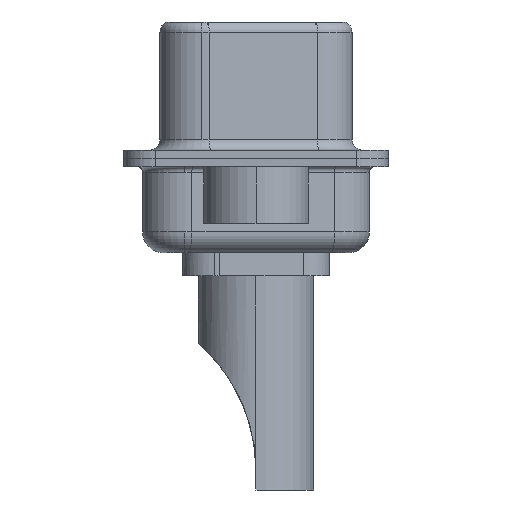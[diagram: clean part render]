
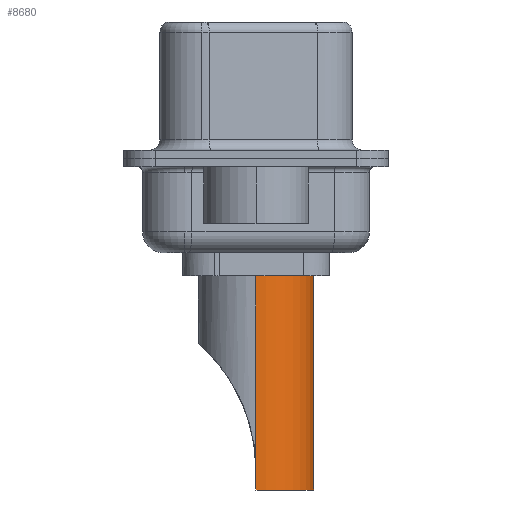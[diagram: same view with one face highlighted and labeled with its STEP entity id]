
A CAD part, left-side view. The second image highlights one B-rep face of the part: STEP entity #8680.
In plain terms, the highlighted cylindrical face has radius 2.75 mm (diameter 5.5 mm), a partial arc.
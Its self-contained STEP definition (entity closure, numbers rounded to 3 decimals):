
#60 = ORIENTED_EDGE ( 'NONE', *, *, #17279, .F. ) ;
#1039 = EDGE_CURVE ( 'NONE', #5639, #16368, #12568, .T. ) ;
#1148 = DIRECTION ( 'NONE',  ( 0., 0., 1. ) ) ;
#1777 = AXIS2_PLACEMENT_3D ( 'NONE', #18766, #11845, #2137 ) ;
#1958 = CARTESIAN_POINT ( 'NONE',  ( -2.75, 0., -7.764 ) ) ;
#2102 = CARTESIAN_POINT ( 'NONE',  ( 2.75, 0., 4.234 ) ) ;
#2137 = DIRECTION ( 'NONE',  ( 1., 0., 0. ) ) ;
#2192 = VERTEX_POINT ( 'NONE', #9690 ) ;
#2249 = ORIENTED_EDGE ( 'NONE', *, *, #11430, .F. ) ;
#2395 = ORIENTED_EDGE ( 'NONE', *, *, #1039, .T. ) ;
#2445 = EDGE_CURVE ( 'NONE', #2192, #6713, #10845, .T. ) ;
#2940 = EDGE_CURVE ( 'NONE', #2192, #16368, #4265, .T. ) ;
#3473 = DIRECTION ( 'NONE',  ( 0., 0., -1. ) ) ;
#4077 = CARTESIAN_POINT ( 'NONE',  ( 0., 0., -8.7 ) ) ;
#4265 = LINE ( 'NONE', #4713, #15809 ) ;
#4396 = DIRECTION ( 'NONE',  ( 0., 0., 1. ) ) ;
#4713 = CARTESIAN_POINT ( 'NONE',  ( 2.75, 0., -8.7 ) ) ;
#4761 = CARTESIAN_POINT ( 'NONE',  ( 2.75, 0., 1.5 ) ) ;
#5161 = VECTOR ( 'NONE', #11260, 1000. ) ;
#5171 = DIRECTION ( 'NONE',  ( 1., 0., 0. ) ) ;
#5639 = VERTEX_POINT ( 'NONE', #11441 ) ;
#5860 = DIRECTION ( 'NONE',  ( 1., 0., 0. ) ) ;
#6185 = EDGE_LOOP ( 'NONE', ( #60, #14932, #2395, #10513, #18030, #2249 ) ) ;
#6713 = VERTEX_POINT ( 'NONE', #4761 ) ;
#6759 = AXIS2_PLACEMENT_3D ( 'NONE', #11242, #18667, #5171 ) ;
#6827 = VECTOR ( 'NONE', #10425, 1000. ) ;
#7503 = CIRCLE ( 'NONE', #6759, 2.75 ) ;
#8680 = ADVANCED_FACE ( 'NONE', ( #13974 ), #19403, .T. ) ;
#9370 = AXIS2_PLACEMENT_3D ( 'NONE', #4077, #4396, #5860 ) ;
#9690 = CARTESIAN_POINT ( 'NONE',  ( 2.75, 0., -7.764 ) ) ;
#10027 = CARTESIAN_POINT ( 'NONE',  ( -2.75, 0., 4.234 ) ) ;
#10425 = DIRECTION ( 'NONE',  ( 0., 0., 1. ) ) ;
#10513 = ORIENTED_EDGE ( 'NONE', *, *, #2940, .F. ) ;
#10845 = LINE ( 'NONE', #2102, #6827 ) ;
#11242 = CARTESIAN_POINT ( 'NONE',  ( 0., 0., 1.5 ) ) ;
#11260 = DIRECTION ( 'NONE',  ( 0., 0., -1. ) ) ;
#11430 = EDGE_CURVE ( 'NONE', #19466, #6713, #7503, .T. ) ;
#11441 = CARTESIAN_POINT ( 'NONE',  ( -2.75, 0., -8.7 ) ) ;
#11449 = CARTESIAN_POINT ( 'NONE',  ( -2.75, 0., -8.7 ) ) ;
#11845 = DIRECTION ( 'NONE',  ( 0., 0., 1. ) ) ;
#12568 = CIRCLE ( 'NONE', #9370, 2.75 ) ;
#13974 = FACE_OUTER_BOUND ( 'NONE', #6185, .T. ) ;
#14932 = ORIENTED_EDGE ( 'NONE', *, *, #15976, .T. ) ;
#15188 = VERTEX_POINT ( 'NONE', #1958 ) ;
#15553 = LINE ( 'NONE', #11449, #5161 ) ;
#15809 = VECTOR ( 'NONE', #3473, 1000. ) ;
#15976 = EDGE_CURVE ( 'NONE', #15188, #5639, #15553, .T. ) ;
#16106 = LINE ( 'NONE', #10027, #18440 ) ;
#16368 = VERTEX_POINT ( 'NONE', #16379 ) ;
#16379 = CARTESIAN_POINT ( 'NONE',  ( 2.75, 0., -8.7 ) ) ;
#17279 = EDGE_CURVE ( 'NONE', #15188, #19466, #16106, .T. ) ;
#18030 = ORIENTED_EDGE ( 'NONE', *, *, #2445, .T. ) ;
#18440 = VECTOR ( 'NONE', #1148, 1000. ) ;
#18667 = DIRECTION ( 'NONE',  ( 0., 0., 1. ) ) ;
#18766 = CARTESIAN_POINT ( 'NONE',  ( 0., 0., 4.234 ) ) ;
#18952 = CARTESIAN_POINT ( 'NONE',  ( -2.75, 0., 1.5 ) ) ;
#19403 = CYLINDRICAL_SURFACE ( 'NONE', #1777, 2.75 ) ;
#19466 = VERTEX_POINT ( 'NONE', #18952 ) ;
